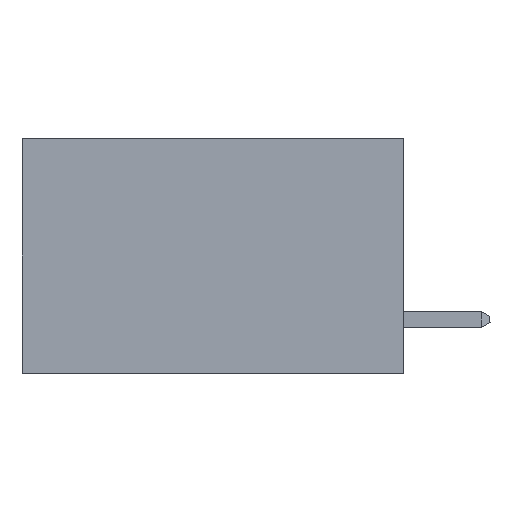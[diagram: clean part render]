
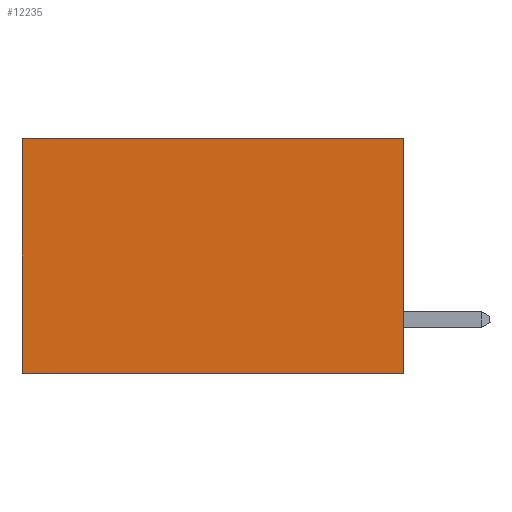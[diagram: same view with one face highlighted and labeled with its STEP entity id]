
A CAD part, left-side view. The second image highlights one B-rep face of the part: STEP entity #12235.
In plain terms, the highlighted planar face has unit normal (-1, 0, 0).
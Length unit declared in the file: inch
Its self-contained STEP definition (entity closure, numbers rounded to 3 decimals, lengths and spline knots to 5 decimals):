
#805 = VERTEX_POINT ( 'NONE', #14180 ) ;
#909 = CARTESIAN_POINT ( 'NONE',  ( 0.2875, 0.6, -0.37 ) ) ;
#3054 = VECTOR ( 'NONE', #26002, 39.37008 ) ;
#3321 = EDGE_CURVE ( 'NONE', #805, #20153, #24235, .T. ) ;
#3714 = CARTESIAN_POINT ( 'NONE',  ( 0.2875, 0., 0. ) ) ;
#6884 = EDGE_LOOP ( 'NONE', ( #8666, #31803, #8890, #8531 ) ) ;
#8390 = PLANE ( 'NONE',  #16704 ) ;
#8531 = ORIENTED_EDGE ( 'NONE', *, *, #13017, .T. ) ;
#8666 = ORIENTED_EDGE ( 'NONE', *, *, #3321, .T. ) ;
#8890 = ORIENTED_EDGE ( 'NONE', *, *, #17333, .F. ) ;
#9227 = VECTOR ( 'NONE', #30963, 39.37008 ) ;
#10403 = FACE_OUTER_BOUND ( 'NONE', #6884, .T. ) ;
#10737 = LINE ( 'NONE', #3714, #20746 ) ;
#12074 = CARTESIAN_POINT ( 'NONE',  ( 0.2875, 0., 0. ) ) ;
#12235 = ADVANCED_FACE ( 'NONE', ( #10403 ), #8390, .F. ) ;
#13017 = EDGE_CURVE ( 'NONE', #34236, #805, #10737, .T. ) ;
#14180 = CARTESIAN_POINT ( 'NONE',  ( 0.2875, 0.6, 0. ) ) ;
#16704 = AXIS2_PLACEMENT_3D ( 'NONE', #23869, #21644, #26559 ) ;
#17011 = VECTOR ( 'NONE', #28995, 39.37008 ) ;
#17333 = EDGE_CURVE ( 'NONE', #34236, #24903, #25087, .T. ) ;
#17827 = CARTESIAN_POINT ( 'NONE',  ( 0.2875, 0., 0. ) ) ;
#17848 = LINE ( 'NONE', #34253, #17011 ) ;
#20153 = VERTEX_POINT ( 'NONE', #909 ) ;
#20746 = VECTOR ( 'NONE', #22289, 39.37008 ) ;
#21644 = DIRECTION ( 'NONE',  ( 1., 0., 0. ) ) ;
#22289 = DIRECTION ( 'NONE',  ( 0., 1., 0. ) ) ;
#23697 = CARTESIAN_POINT ( 'NONE',  ( 0.2875, 0., -0.37 ) ) ;
#23869 = CARTESIAN_POINT ( 'NONE',  ( 0.2875, 0., 0. ) ) ;
#24235 = LINE ( 'NONE', #28654, #3054 ) ;
#24903 = VERTEX_POINT ( 'NONE', #23697 ) ;
#25087 = LINE ( 'NONE', #12074, #9227 ) ;
#26002 = DIRECTION ( 'NONE',  ( 0., 0., -1. ) ) ;
#26559 = DIRECTION ( 'NONE',  ( 0., 0., -1. ) ) ;
#28654 = CARTESIAN_POINT ( 'NONE',  ( 0.2875, 0.6, 0. ) ) ;
#28995 = DIRECTION ( 'NONE',  ( 0., 1., 0. ) ) ;
#29680 = EDGE_CURVE ( 'NONE', #24903, #20153, #17848, .T. ) ;
#30963 = DIRECTION ( 'NONE',  ( 0., 0., -1. ) ) ;
#31803 = ORIENTED_EDGE ( 'NONE', *, *, #29680, .F. ) ;
#34236 = VERTEX_POINT ( 'NONE', #17827 ) ;
#34253 = CARTESIAN_POINT ( 'NONE',  ( 0.2875, 0., -0.37 ) ) ;
